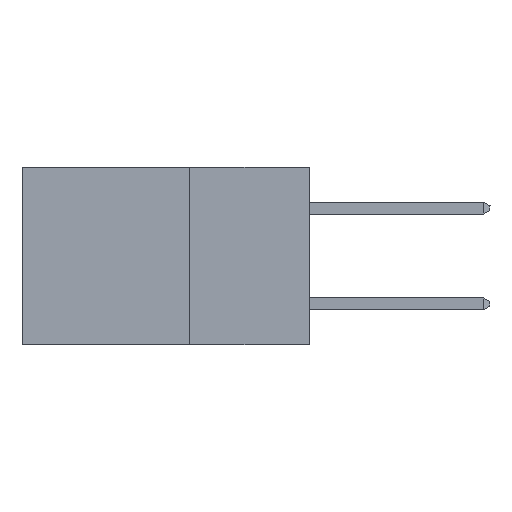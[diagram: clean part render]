
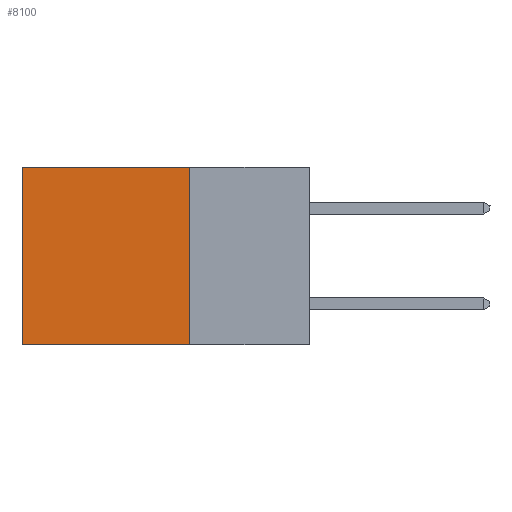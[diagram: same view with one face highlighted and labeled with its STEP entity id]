
A CAD part, left-side view. The second image highlights one B-rep face of the part: STEP entity #8100.
In plain terms, the highlighted planar face has unit normal (-1, 0, 0).
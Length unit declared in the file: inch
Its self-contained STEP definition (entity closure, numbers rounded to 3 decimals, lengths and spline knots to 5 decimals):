
#692 = VERTEX_POINT ( 'NONE', #11537 ) ;
#1155 = AXIS2_PLACEMENT_3D ( 'NONE', #1352, #2668, #11664 ) ;
#1352 = CARTESIAN_POINT ( 'NONE',  ( 0.2875, 0.25, 0. ) ) ;
#2298 = EDGE_CURVE ( 'NONE', #12010, #13805, #8545, .T. ) ;
#2668 = DIRECTION ( 'NONE',  ( 1., 0., 0. ) ) ;
#2857 = DIRECTION ( 'NONE',  ( 0., 1., 0. ) ) ;
#2990 = VECTOR ( 'NONE', #13126, 39.37008 ) ;
#3400 = LINE ( 'NONE', #11856, #2990 ) ;
#4853 = CARTESIAN_POINT ( 'NONE',  ( 0.2875, 0.6, 0. ) ) ;
#5108 = VECTOR ( 'NONE', #5288, 39.37008 ) ;
#5159 = EDGE_CURVE ( 'NONE', #13805, #15992, #6972, .T. ) ;
#5288 = DIRECTION ( 'NONE',  ( 0., 1., 0. ) ) ;
#5482 = LINE ( 'NONE', #10573, #15703 ) ;
#6462 = EDGE_LOOP ( 'NONE', ( #7370, #7398, #7537, #7555 ) ) ;
#6972 = LINE ( 'NONE', #16516, #13353 ) ;
#7370 = ORIENTED_EDGE ( 'NONE', *, *, #5159, .T. ) ;
#7398 = ORIENTED_EDGE ( 'NONE', *, *, #8870, .F. ) ;
#7537 = ORIENTED_EDGE ( 'NONE', *, *, #15540, .F. ) ;
#7555 = ORIENTED_EDGE ( 'NONE', *, *, #2298, .T. ) ;
#7597 = DIRECTION ( 'NONE',  ( 0., 0., -1. ) ) ;
#8100 = ADVANCED_FACE ( 'NONE', ( #10320 ), #10379, .F. ) ;
#8545 = LINE ( 'NONE', #9364, #5108 ) ;
#8870 = EDGE_CURVE ( 'NONE', #692, #15992, #5482, .T. ) ;
#9364 = CARTESIAN_POINT ( 'NONE',  ( 0.2875, 0.25, 0. ) ) ;
#9899 = CARTESIAN_POINT ( 'NONE',  ( 0.2875, 0.25, 0. ) ) ;
#10320 = FACE_OUTER_BOUND ( 'NONE', #6462, .T. ) ;
#10379 = PLANE ( 'NONE',  #1155 ) ;
#10573 = CARTESIAN_POINT ( 'NONE',  ( 0.2875, 0.25, -0.37 ) ) ;
#11537 = CARTESIAN_POINT ( 'NONE',  ( 0.2875, 0.25, -0.37 ) ) ;
#11664 = DIRECTION ( 'NONE',  ( 0., 0., -1. ) ) ;
#11856 = CARTESIAN_POINT ( 'NONE',  ( 0.2875, 0.25, 0. ) ) ;
#12010 = VERTEX_POINT ( 'NONE', #9899 ) ;
#13126 = DIRECTION ( 'NONE',  ( 0., 0., -1. ) ) ;
#13353 = VECTOR ( 'NONE', #7597, 39.37008 ) ;
#13805 = VERTEX_POINT ( 'NONE', #4853 ) ;
#15233 = CARTESIAN_POINT ( 'NONE',  ( 0.2875, 0.6, -0.37 ) ) ;
#15540 = EDGE_CURVE ( 'NONE', #12010, #692, #3400, .T. ) ;
#15703 = VECTOR ( 'NONE', #2857, 39.37008 ) ;
#15992 = VERTEX_POINT ( 'NONE', #15233 ) ;
#16516 = CARTESIAN_POINT ( 'NONE',  ( 0.2875, 0.6, 0. ) ) ;
